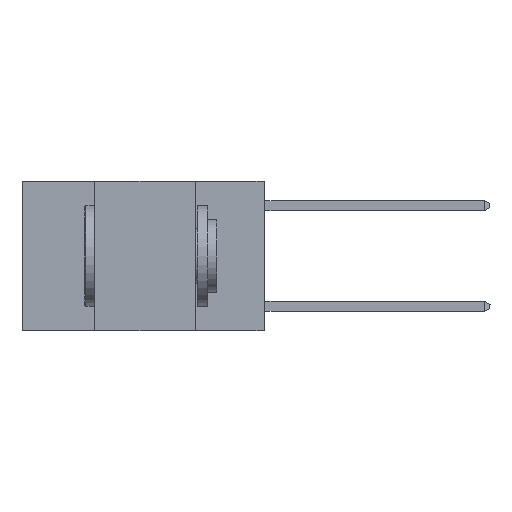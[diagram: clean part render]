
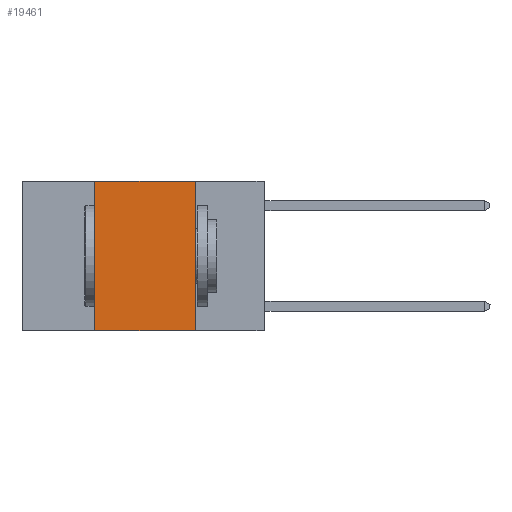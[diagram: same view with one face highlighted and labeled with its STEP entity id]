
A CAD part, left-side view. The second image highlights one B-rep face of the part: STEP entity #19461.
In plain terms, the highlighted planar face has unit normal (-1, 0, 0).
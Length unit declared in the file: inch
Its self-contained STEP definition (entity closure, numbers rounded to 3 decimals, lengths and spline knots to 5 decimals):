
#312 = VECTOR ( 'NONE', #23466, 39.37008 ) ;
#563 = EDGE_CURVE ( 'NONE', #8271, #22261, #17784, .T. ) ;
#1371 = DIRECTION ( 'NONE',  ( 0., 0., -1. ) ) ;
#2509 = DIRECTION ( 'NONE',  ( 0., 0., -1. ) ) ;
#2749 = ORIENTED_EDGE ( 'NONE', *, *, #12984, .F. ) ;
#5950 = AXIS2_PLACEMENT_3D ( 'NONE', #9368, #16315, #2509 ) ;
#6747 = CARTESIAN_POINT ( 'NONE',  ( 0., 0.42, -0.37 ) ) ;
#7231 = VERTEX_POINT ( 'NONE', #6747 ) ;
#8140 = ORIENTED_EDGE ( 'NONE', *, *, #563, .F. ) ;
#8271 = VERTEX_POINT ( 'NONE', #8516 ) ;
#8516 = CARTESIAN_POINT ( 'NONE',  ( 0., 0.17, 0. ) ) ;
#8519 = VECTOR ( 'NONE', #21718, 39.37008 ) ;
#8864 = ORIENTED_EDGE ( 'NONE', *, *, #11023, .F. ) ;
#9051 = LINE ( 'NONE', #11649, #14488 ) ;
#9368 = CARTESIAN_POINT ( 'NONE',  ( 0., 0.6, 0. ) ) ;
#9589 = ORIENTED_EDGE ( 'NONE', *, *, #16914, .T. ) ;
#9662 = CARTESIAN_POINT ( 'NONE',  ( 0., 0.42, 0. ) ) ;
#11023 = EDGE_CURVE ( 'NONE', #7231, #11800, #17949, .T. ) ;
#11189 = CARTESIAN_POINT ( 'NONE',  ( 0., 0.17, -0.37 ) ) ;
#11649 = CARTESIAN_POINT ( 'NONE',  ( 0., 0.6, -0.37 ) ) ;
#11800 = VERTEX_POINT ( 'NONE', #12077 ) ;
#12077 = CARTESIAN_POINT ( 'NONE',  ( 0., 0.42, 0. ) ) ;
#12602 = CARTESIAN_POINT ( 'NONE',  ( 0., 0.6, 0. ) ) ;
#12984 = EDGE_CURVE ( 'NONE', #11800, #8271, #26235, .T. ) ;
#14488 = VECTOR ( 'NONE', #18451, 39.37008 ) ;
#14827 = EDGE_LOOP ( 'NONE', ( #8140, #2749, #8864, #9589 ) ) ;
#16315 = DIRECTION ( 'NONE',  ( 1., 0., 0. ) ) ;
#16914 = EDGE_CURVE ( 'NONE', #7231, #22261, #9051, .T. ) ;
#17784 = LINE ( 'NONE', #23920, #23196 ) ;
#17949 = LINE ( 'NONE', #9662, #312 ) ;
#18451 = DIRECTION ( 'NONE',  ( 0., -1., 0. ) ) ;
#19461 = ADVANCED_FACE ( 'NONE', ( #22035 ), #23164, .F. ) ;
#21718 = DIRECTION ( 'NONE',  ( 0., -1., 0. ) ) ;
#22035 = FACE_OUTER_BOUND ( 'NONE', #14827, .T. ) ;
#22261 = VERTEX_POINT ( 'NONE', #11189 ) ;
#23164 = PLANE ( 'NONE',  #5950 ) ;
#23196 = VECTOR ( 'NONE', #1371, 39.37008 ) ;
#23466 = DIRECTION ( 'NONE',  ( 0., 0., 1. ) ) ;
#23920 = CARTESIAN_POINT ( 'NONE',  ( 0., 0.17, 0. ) ) ;
#26235 = LINE ( 'NONE', #12602, #8519 ) ;
